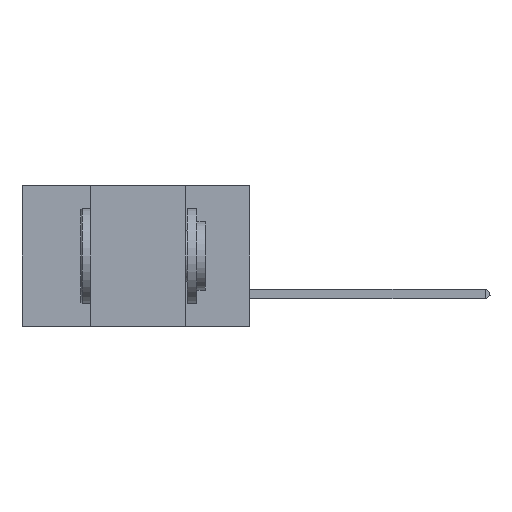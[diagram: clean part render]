
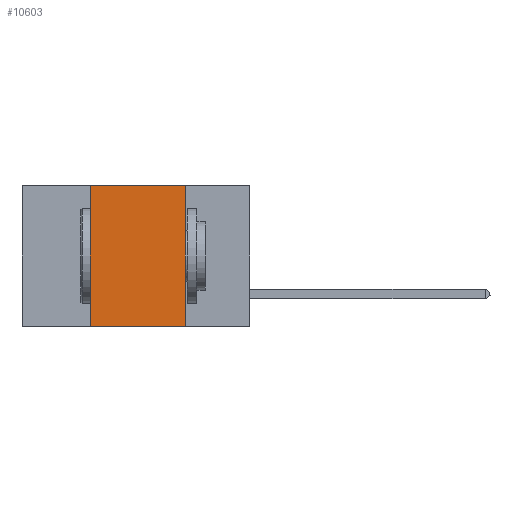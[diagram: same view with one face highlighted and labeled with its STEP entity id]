
A CAD part, left-side view. The second image highlights one B-rep face of the part: STEP entity #10603.
In plain terms, the highlighted planar face has unit normal (-1, 0, 0).
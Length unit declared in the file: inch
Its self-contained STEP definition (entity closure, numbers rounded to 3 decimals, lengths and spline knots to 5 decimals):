
#1205 = VERTEX_POINT ( 'NONE', #38436 ) ;
#1915 = EDGE_LOOP ( 'NONE', ( #36200, #9335, #36830, #17677 ) ) ;
#4037 = DIRECTION ( 'NONE',  ( 0., 0., 1. ) ) ;
#4288 = LINE ( 'NONE', #29252, #30677 ) ;
#7638 = FACE_OUTER_BOUND ( 'NONE', #1915, .T. ) ;
#8189 = PLANE ( 'NONE',  #26757 ) ;
#9335 = ORIENTED_EDGE ( 'NONE', *, *, #23828, .F. ) ;
#10603 = ADVANCED_FACE ( 'NONE', ( #7638 ), #8189, .F. ) ;
#13748 = CARTESIAN_POINT ( 'NONE',  ( 0., 0.17, -0.37 ) ) ;
#14673 = DIRECTION ( 'NONE',  ( 0., -1., 0. ) ) ;
#16258 = EDGE_CURVE ( 'NONE', #28269, #26425, #16772, .T. ) ;
#16772 = LINE ( 'NONE', #35367, #34871 ) ;
#17677 = ORIENTED_EDGE ( 'NONE', *, *, #22169, .T. ) ;
#21130 = VECTOR ( 'NONE', #32233, 39.37008 ) ;
#22169 = EDGE_CURVE ( 'NONE', #31615, #26425, #4288, .T. ) ;
#23828 = EDGE_CURVE ( 'NONE', #1205, #28269, #42153, .T. ) ;
#25858 = CARTESIAN_POINT ( 'NONE',  ( 0., 0.42, 0. ) ) ;
#26425 = VERTEX_POINT ( 'NONE', #13748 ) ;
#26565 = DIRECTION ( 'NONE',  ( 1., 0., 0. ) ) ;
#26757 = AXIS2_PLACEMENT_3D ( 'NONE', #37901, #26565, #45633 ) ;
#28269 = VERTEX_POINT ( 'NONE', #34798 ) ;
#28862 = CARTESIAN_POINT ( 'NONE',  ( 0., 0.6, 0. ) ) ;
#29252 = CARTESIAN_POINT ( 'NONE',  ( 0., 0.6, -0.37 ) ) ;
#30677 = VECTOR ( 'NONE', #14673, 39.37008 ) ;
#31615 = VERTEX_POINT ( 'NONE', #36400 ) ;
#32233 = DIRECTION ( 'NONE',  ( 0., -1., 0. ) ) ;
#34798 = CARTESIAN_POINT ( 'NONE',  ( 0., 0.17, 0. ) ) ;
#34871 = VECTOR ( 'NONE', #42581, 39.37008 ) ;
#35367 = CARTESIAN_POINT ( 'NONE',  ( 0., 0.17, 0. ) ) ;
#36200 = ORIENTED_EDGE ( 'NONE', *, *, #16258, .F. ) ;
#36400 = CARTESIAN_POINT ( 'NONE',  ( 0., 0.42, -0.37 ) ) ;
#36830 = ORIENTED_EDGE ( 'NONE', *, *, #40368, .F. ) ;
#37901 = CARTESIAN_POINT ( 'NONE',  ( 0., 0.6, 0. ) ) ;
#38436 = CARTESIAN_POINT ( 'NONE',  ( 0., 0.42, 0. ) ) ;
#40220 = LINE ( 'NONE', #25858, #44313 ) ;
#40368 = EDGE_CURVE ( 'NONE', #31615, #1205, #40220, .T. ) ;
#42153 = LINE ( 'NONE', #28862, #21130 ) ;
#42581 = DIRECTION ( 'NONE',  ( 0., 0., -1. ) ) ;
#44313 = VECTOR ( 'NONE', #4037, 39.37008 ) ;
#45633 = DIRECTION ( 'NONE',  ( 0., 0., -1. ) ) ;
